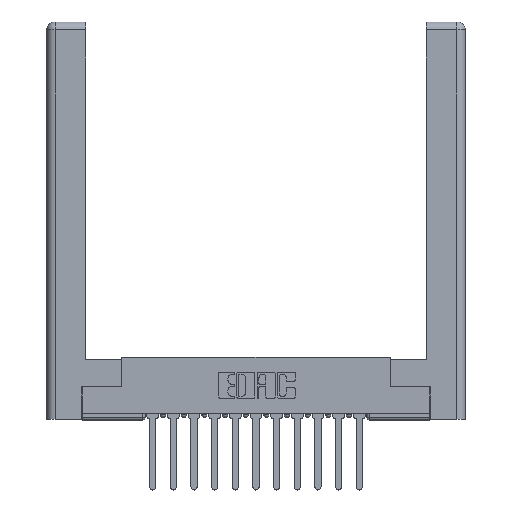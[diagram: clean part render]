
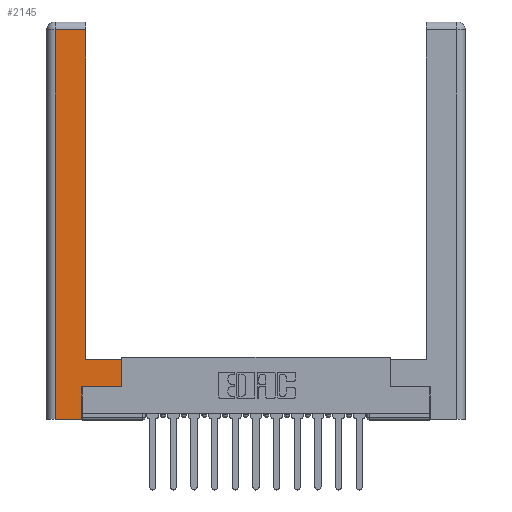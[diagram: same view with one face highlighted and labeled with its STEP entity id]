
A CAD part, top view. The second image highlights one B-rep face of the part: STEP entity #2145.
In plain terms, the highlighted planar face has unit normal (0, 0, 1).
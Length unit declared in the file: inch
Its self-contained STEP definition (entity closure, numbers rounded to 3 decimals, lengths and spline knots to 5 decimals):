
#877 = CARTESIAN_POINT ( 'NONE',  ( 0.295, 0.45, 0. ) ) ;
#1094 = VERTEX_POINT ( 'NONE', #5836 ) ;
#1167 = CARTESIAN_POINT ( 'NONE',  ( 0.0615, 2.94, 0. ) ) ;
#1206 = CARTESIAN_POINT ( 'NONE',  ( 0.295, 3., 0. ) ) ;
#1290 = VECTOR ( 'NONE', #13182, 39.37008 ) ;
#1516 = CARTESIAN_POINT ( 'NONE',  ( 0.295, 0.45, 0. ) ) ;
#2028 = LINE ( 'NONE', #877, #12663 ) ;
#2113 = DIRECTION ( 'NONE',  ( -1., 0., 0. ) ) ;
#2145 = ADVANCED_FACE ( 'NONE', ( #9920 ), #14897, .F. ) ;
#2250 = VECTOR ( 'NONE', #7838, 39.37008 ) ;
#2257 = LINE ( 'NONE', #4571, #10630 ) ;
#3215 = ORIENTED_EDGE ( 'NONE', *, *, #4201, .T. ) ;
#3514 = DIRECTION ( 'NONE',  ( 0., 1., 0. ) ) ;
#3657 = DIRECTION ( 'NONE',  ( -1., 0., 0. ) ) ;
#4005 = EDGE_CURVE ( 'NONE', #14632, #6915, #10797, .T. ) ;
#4201 = EDGE_CURVE ( 'NONE', #1094, #11523, #4609, .T. ) ;
#4571 = CARTESIAN_POINT ( 'NONE',  ( 0.565, 0.245, 0. ) ) ;
#4609 = LINE ( 'NONE', #12417, #15956 ) ;
#5772 = CARTESIAN_POINT ( 'NONE',  ( 0.565, 0.245, 0. ) ) ;
#5836 = CARTESIAN_POINT ( 'NONE',  ( 0.0615, 0., 0. ) ) ;
#6101 = ORIENTED_EDGE ( 'NONE', *, *, #4005, .T. ) ;
#6123 = ORIENTED_EDGE ( 'NONE', *, *, #9741, .T. ) ;
#6166 = VERTEX_POINT ( 'NONE', #10544 ) ;
#6203 = CARTESIAN_POINT ( 'NONE',  ( 0., 0., 0. ) ) ;
#6621 = EDGE_CURVE ( 'NONE', #6166, #14879, #14813, .T. ) ;
#6915 = VERTEX_POINT ( 'NONE', #11788 ) ;
#7330 = DIRECTION ( 'NONE',  ( 1., 0., 0. ) ) ;
#7656 = AXIS2_PLACEMENT_3D ( 'NONE', #6203, #8430, #3657 ) ;
#7815 = ORIENTED_EDGE ( 'NONE', *, *, #14930, .T. ) ;
#7838 = DIRECTION ( 'NONE',  ( 0., 1., 0. ) ) ;
#8354 = VECTOR ( 'NONE', #11781, 39.37008 ) ;
#8430 = DIRECTION ( 'NONE',  ( 0., 0., -1. ) ) ;
#8984 = CARTESIAN_POINT ( 'NONE',  ( 0.0615, 0., 0. ) ) ;
#9249 = CARTESIAN_POINT ( 'NONE',  ( 0.265, 0.245, 0. ) ) ;
#9353 = ORIENTED_EDGE ( 'NONE', *, *, #11409, .T. ) ;
#9478 = CARTESIAN_POINT ( 'NONE',  ( 0.565, 0.45, 0. ) ) ;
#9594 = DIRECTION ( 'NONE',  ( 1., 0., 0. ) ) ;
#9741 = EDGE_CURVE ( 'NONE', #6915, #12894, #2028, .T. ) ;
#9920 = FACE_OUTER_BOUND ( 'NONE', #16195, .T. ) ;
#10145 = ORIENTED_EDGE ( 'NONE', *, *, #14521, .T. ) ;
#10394 = LINE ( 'NONE', #8984, #12233 ) ;
#10544 = CARTESIAN_POINT ( 'NONE',  ( 0.295, 2.94, 0. ) ) ;
#10630 = VECTOR ( 'NONE', #9594, 39.37008 ) ;
#10797 = LINE ( 'NONE', #9478, #8354 ) ;
#10987 = CARTESIAN_POINT ( 'NONE',  ( 0.265, 0.245, 0. ) ) ;
#11409 = EDGE_CURVE ( 'NONE', #13279, #14632, #2257, .T. ) ;
#11523 = VERTEX_POINT ( 'NONE', #12055 ) ;
#11775 = ORIENTED_EDGE ( 'NONE', *, *, #6621, .T. ) ;
#11781 = DIRECTION ( 'NONE',  ( 0., 1., 0. ) ) ;
#11788 = CARTESIAN_POINT ( 'NONE',  ( 0.565, 0.45, 0. ) ) ;
#12055 = CARTESIAN_POINT ( 'NONE',  ( 0.265, 0., 0. ) ) ;
#12233 = VECTOR ( 'NONE', #15369, 39.37008 ) ;
#12417 = CARTESIAN_POINT ( 'NONE',  ( 0.265, 0., 0. ) ) ;
#12663 = VECTOR ( 'NONE', #2113, 39.37008 ) ;
#12894 = VERTEX_POINT ( 'NONE', #1516 ) ;
#12935 = LINE ( 'NONE', #9249, #2250 ) ;
#13182 = DIRECTION ( 'NONE',  ( -1., 0., 0. ) ) ;
#13279 = VERTEX_POINT ( 'NONE', #10987 ) ;
#14521 = EDGE_CURVE ( 'NONE', #11523, #13279, #12935, .T. ) ;
#14632 = VERTEX_POINT ( 'NONE', #5772 ) ;
#14813 = LINE ( 'NONE', #15963, #1290 ) ;
#14879 = VERTEX_POINT ( 'NONE', #1167 ) ;
#14897 = PLANE ( 'NONE',  #7656 ) ;
#14915 = LINE ( 'NONE', #1206, #15128 ) ;
#14930 = EDGE_CURVE ( 'NONE', #14879, #1094, #10394, .T. ) ;
#15128 = VECTOR ( 'NONE', #3514, 39.37008 ) ;
#15369 = DIRECTION ( 'NONE',  ( 0., -1., 0. ) ) ;
#15700 = EDGE_CURVE ( 'NONE', #12894, #6166, #14915, .T. ) ;
#15956 = VECTOR ( 'NONE', #7330, 39.37008 ) ;
#15963 = CARTESIAN_POINT ( 'NONE',  ( 0.0615, 2.94, 0. ) ) ;
#16186 = ORIENTED_EDGE ( 'NONE', *, *, #15700, .T. ) ;
#16195 = EDGE_LOOP ( 'NONE', ( #16186, #11775, #7815, #3215, #10145, #9353, #6101, #6123 ) ) ;
